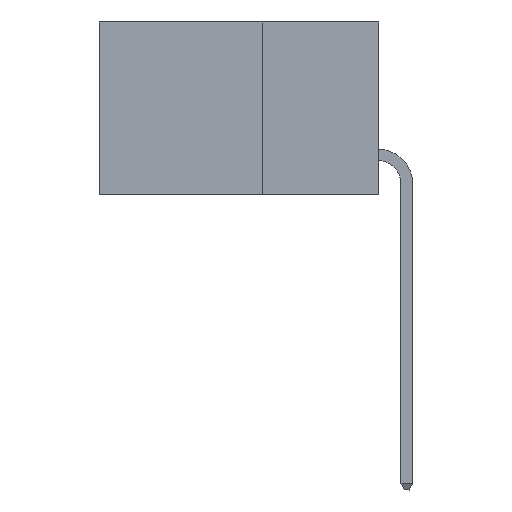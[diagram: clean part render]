
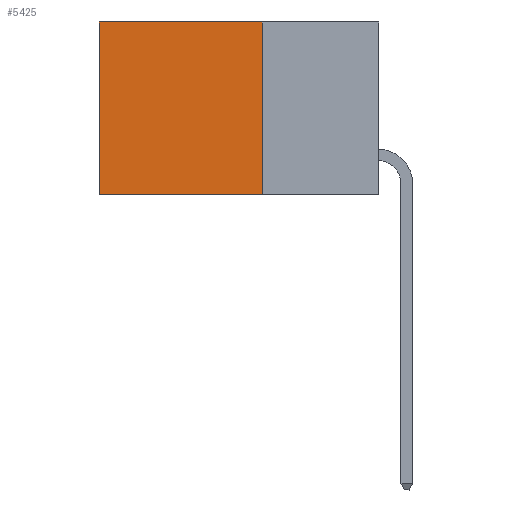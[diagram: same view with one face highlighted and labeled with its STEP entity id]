
A CAD part, left-side view. The second image highlights one B-rep face of the part: STEP entity #5425.
In plain terms, the highlighted planar face has unit normal (-1, 0, 0).
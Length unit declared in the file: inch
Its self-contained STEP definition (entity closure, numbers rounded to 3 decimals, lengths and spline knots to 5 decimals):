
#166 = CARTESIAN_POINT ( 'NONE',  ( 0.298, 0.25, -0.37 ) ) ;
#571 = DIRECTION ( 'NONE',  ( 0., 1., 0. ) ) ;
#898 = ORIENTED_EDGE ( 'NONE', *, *, #2210, .T. ) ;
#1065 = VERTEX_POINT ( 'NONE', #4141 ) ;
#1428 = DIRECTION ( 'NONE',  ( 0., 0., -1. ) ) ;
#1463 = DIRECTION ( 'NONE',  ( 0., 0., -1. ) ) ;
#1489 = VECTOR ( 'NONE', #571, 39.37008 ) ;
#1841 = ORIENTED_EDGE ( 'NONE', *, *, #7472, .F. ) ;
#1978 = EDGE_CURVE ( 'NONE', #1065, #4785, #6006, .T. ) ;
#2091 = AXIS2_PLACEMENT_3D ( 'NONE', #4541, #6515, #1428 ) ;
#2210 = EDGE_CURVE ( 'NONE', #6486, #4889, #9891, .T. ) ;
#2330 = EDGE_LOOP ( 'NONE', ( #9109, #7564, #1841, #898 ) ) ;
#3688 = PLANE ( 'NONE',  #2091 ) ;
#4055 = FACE_OUTER_BOUND ( 'NONE', #2330, .T. ) ;
#4141 = CARTESIAN_POINT ( 'NONE',  ( 0.298, 0.25, -0.37 ) ) ;
#4144 = DIRECTION ( 'NONE',  ( 0., 0., -1. ) ) ;
#4407 = VECTOR ( 'NONE', #7751, 39.37008 ) ;
#4541 = CARTESIAN_POINT ( 'NONE',  ( 0.298, 0.25, 0. ) ) ;
#4785 = VERTEX_POINT ( 'NONE', #6377 ) ;
#4889 = VERTEX_POINT ( 'NONE', #6605 ) ;
#5425 = ADVANCED_FACE ( 'NONE', ( #4055 ), #3688, .F. ) ;
#5541 = CARTESIAN_POINT ( 'NONE',  ( 0.298, 0.25, 0. ) ) ;
#5593 = LINE ( 'NONE', #9243, #8401 ) ;
#6006 = LINE ( 'NONE', #166, #4407 ) ;
#6324 = LINE ( 'NONE', #10935, #11009 ) ;
#6377 = CARTESIAN_POINT ( 'NONE',  ( 0.298, 0.6, -0.37 ) ) ;
#6486 = VERTEX_POINT ( 'NONE', #9599 ) ;
#6515 = DIRECTION ( 'NONE',  ( 1., 0., 0. ) ) ;
#6605 = CARTESIAN_POINT ( 'NONE',  ( 0.298, 0.6, 0. ) ) ;
#7472 = EDGE_CURVE ( 'NONE', #6486, #1065, #6324, .T. ) ;
#7564 = ORIENTED_EDGE ( 'NONE', *, *, #1978, .F. ) ;
#7751 = DIRECTION ( 'NONE',  ( 0., 1., 0. ) ) ;
#8401 = VECTOR ( 'NONE', #4144, 39.37008 ) ;
#9109 = ORIENTED_EDGE ( 'NONE', *, *, #9517, .T. ) ;
#9243 = CARTESIAN_POINT ( 'NONE',  ( 0.298, 0.6, 0. ) ) ;
#9517 = EDGE_CURVE ( 'NONE', #4889, #4785, #5593, .T. ) ;
#9599 = CARTESIAN_POINT ( 'NONE',  ( 0.298, 0.25, 0. ) ) ;
#9891 = LINE ( 'NONE', #5541, #1489 ) ;
#10935 = CARTESIAN_POINT ( 'NONE',  ( 0.298, 0.25, 0. ) ) ;
#11009 = VECTOR ( 'NONE', #1463, 39.37008 ) ;
